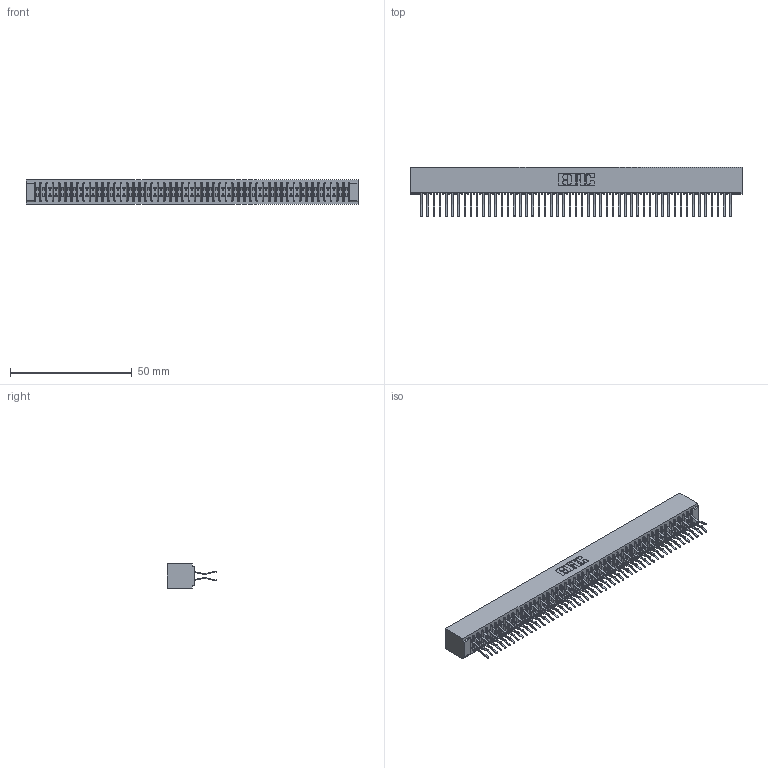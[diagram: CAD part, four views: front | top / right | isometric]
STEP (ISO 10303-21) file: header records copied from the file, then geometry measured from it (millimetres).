
FILE_DESCRIPTION (( 'STEP AP203' ), '1' );
FILE_NAME ('391-102-560-201.STEP', '2018-08-09T20:06:38', ( '' ), ( '' ), 'SwSTEP 2.0', 'SolidWorks 2016', '' );
FILE_SCHEMA (( 'CONFIG_CONTROL_DESIGN' ));
Length unit declared in the file: inch
Products named in the file (3): 341 Part_No Mounting Lugs; 341-292-001_341-292-160; 391-102-560-201
Assembly tree (103 placements, depth 2):
  391-102-560-201
    341 Part_No Mounting Lugs
    341-292-001_341-292-160  x102
Bounding box: 136.53 x 20.37 x 10.16 mm (x, y, z)
Volume: 10426.8 mm3; surface area: 20210.2 mm2
Topology: 103 solids, 103 shells, 7248 faces, 21049 edges, 13654 vertices
Faces by surface type: plane 4144, cylinder 2900, sphere 104, torus 100
Entity records: 60384 total; most frequent: CARTESIAN_POINT 10037, ORIENTED_EDGE 9974, DIRECTION 9737, EDGE_CURVE 4987, VECTOR 4037, LINE 4037, VERTEX_POINT 3150, AXIS2_PLACEMENT_3D 2850
